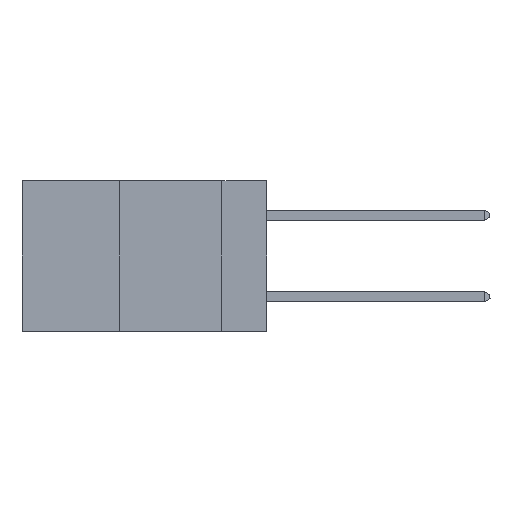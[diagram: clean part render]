
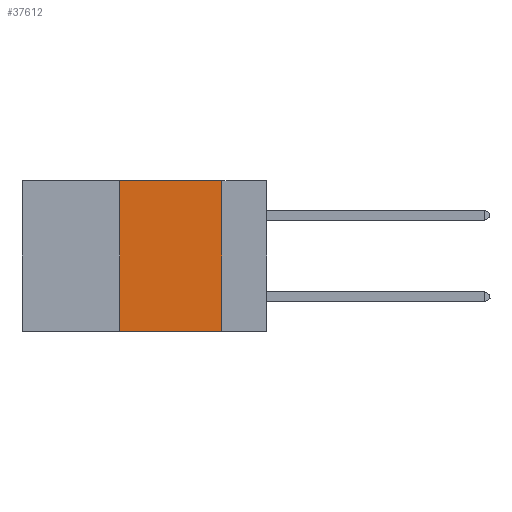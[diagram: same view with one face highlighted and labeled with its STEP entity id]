
A CAD part, left-side view. The second image highlights one B-rep face of the part: STEP entity #37612.
In plain terms, the highlighted planar face has unit normal (-1, 0, 0).
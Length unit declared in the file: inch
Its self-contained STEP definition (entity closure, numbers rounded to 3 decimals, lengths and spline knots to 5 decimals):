
#1179 = AXIS2_PLACEMENT_3D ( 'NONE', #18609, #21865, #36064 ) ;
#1236 = VECTOR ( 'NONE', #22635, 39.37008 ) ;
#1622 = ORIENTED_EDGE ( 'NONE', *, *, #34095, .F. ) ;
#4449 = EDGE_CURVE ( 'NONE', #16629, #41315, #19035, .T. ) ;
#5824 = DIRECTION ( 'NONE',  ( 0., -1., 0. ) ) ;
#6642 = CARTESIAN_POINT ( 'NONE',  ( 0., 0.6, -0.37 ) ) ;
#8810 = ORIENTED_EDGE ( 'NONE', *, *, #4449, .F. ) ;
#9639 = VECTOR ( 'NONE', #5824, 39.37008 ) ;
#10178 = EDGE_LOOP ( 'NONE', ( #8810, #1622, #30540, #29021 ) ) ;
#12097 = FACE_OUTER_BOUND ( 'NONE', #10178, .T. ) ;
#14670 = LINE ( 'NONE', #39212, #37551 ) ;
#15480 = CARTESIAN_POINT ( 'NONE',  ( 0., 0.11, 0. ) ) ;
#16629 = VERTEX_POINT ( 'NONE', #21015 ) ;
#17541 = DIRECTION ( 'NONE',  ( 0., 0., 1. ) ) ;
#18609 = CARTESIAN_POINT ( 'NONE',  ( 0., 0.6, 0. ) ) ;
#18945 = EDGE_CURVE ( 'NONE', #41462, #22065, #14670, .T. ) ;
#19035 = LINE ( 'NONE', #15480, #1236 ) ;
#19224 = VECTOR ( 'NONE', #24418, 39.37008 ) ;
#20884 = CARTESIAN_POINT ( 'NONE',  ( 0., 0.11, -0.37 ) ) ;
#21015 = CARTESIAN_POINT ( 'NONE',  ( 0., 0.11, 0. ) ) ;
#21615 = CARTESIAN_POINT ( 'NONE',  ( 0., 0.36, 0. ) ) ;
#21865 = DIRECTION ( 'NONE',  ( 1., 0., 0. ) ) ;
#22065 = VERTEX_POINT ( 'NONE', #21615 ) ;
#22635 = DIRECTION ( 'NONE',  ( 0., 0., -1. ) ) ;
#24418 = DIRECTION ( 'NONE',  ( 0., -1., 0. ) ) ;
#25204 = CARTESIAN_POINT ( 'NONE',  ( 0., 0.36, -0.37 ) ) ;
#26657 = EDGE_CURVE ( 'NONE', #41462, #41315, #45413, .T. ) ;
#29021 = ORIENTED_EDGE ( 'NONE', *, *, #26657, .T. ) ;
#30540 = ORIENTED_EDGE ( 'NONE', *, *, #18945, .F. ) ;
#34095 = EDGE_CURVE ( 'NONE', #22065, #16629, #42004, .T. ) ;
#34223 = CARTESIAN_POINT ( 'NONE',  ( 0., 0.6, 0. ) ) ;
#36064 = DIRECTION ( 'NONE',  ( 0., 0., -1. ) ) ;
#37551 = VECTOR ( 'NONE', #17541, 39.37008 ) ;
#37612 = ADVANCED_FACE ( 'NONE', ( #12097 ), #40269, .F. ) ;
#39212 = CARTESIAN_POINT ( 'NONE',  ( 0., 0.36, 0. ) ) ;
#40269 = PLANE ( 'NONE',  #1179 ) ;
#41315 = VERTEX_POINT ( 'NONE', #20884 ) ;
#41462 = VERTEX_POINT ( 'NONE', #25204 ) ;
#42004 = LINE ( 'NONE', #34223, #9639 ) ;
#45413 = LINE ( 'NONE', #6642, #19224 ) ;
